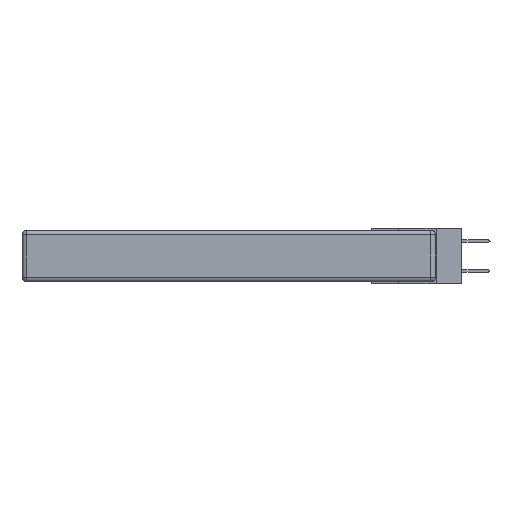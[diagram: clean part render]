
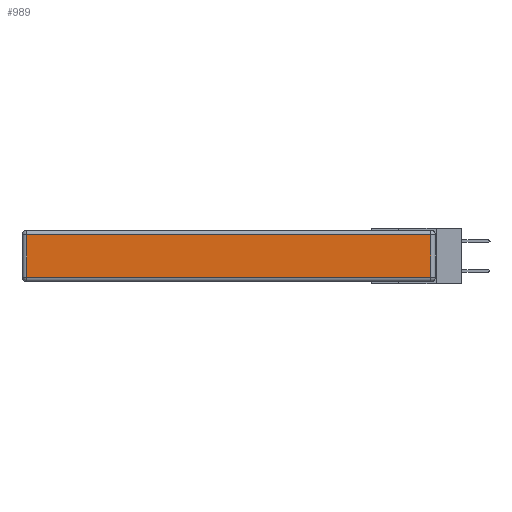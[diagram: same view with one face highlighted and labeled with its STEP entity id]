
A CAD part, left-side view. The second image highlights one B-rep face of the part: STEP entity #989.
In plain terms, the highlighted planar face has unit normal (-1, 0, 0).
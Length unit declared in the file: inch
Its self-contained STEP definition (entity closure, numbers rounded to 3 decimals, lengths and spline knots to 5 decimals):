
#612 = EDGE_CURVE ( 'NONE', #9222, #27523, #4498, .T. ) ;
#835 = CARTESIAN_POINT ( 'NONE',  ( 0., 0., -0.343 ) ) ;
#989 = ADVANCED_FACE ( 'NONE', ( #16311 ), #11534, .T. ) ;
#2759 = CARTESIAN_POINT ( 'NONE',  ( 0., 0., -0.313 ) ) ;
#4498 = LINE ( 'NONE', #10160, #17363 ) ;
#4716 = ORIENTED_EDGE ( 'NONE', *, *, #22027, .T. ) ;
#5216 = DIRECTION ( 'NONE',  ( 0., 0., 1. ) ) ;
#5951 = ORIENTED_EDGE ( 'NONE', *, *, #17439, .T. ) ;
#5953 = CARTESIAN_POINT ( 'NONE',  ( 0., 0.03, -0.03 ) ) ;
#6062 = CARTESIAN_POINT ( 'NONE',  ( 0., 2.75, -0.03 ) ) ;
#6130 = DIRECTION ( 'NONE',  ( 0., 0., 1. ) ) ;
#7300 = CARTESIAN_POINT ( 'NONE',  ( 0., 0.03, -0.313 ) ) ;
#7543 = VECTOR ( 'NONE', #14120, 39.37008 ) ;
#8411 = CARTESIAN_POINT ( 'NONE',  ( 0., 2.72, -0.313 ) ) ;
#8640 = EDGE_CURVE ( 'NONE', #15435, #14206, #14609, .T. ) ;
#8843 = VECTOR ( 'NONE', #10572, 39.37008 ) ;
#9222 = VERTEX_POINT ( 'NONE', #7300 ) ;
#9457 = LINE ( 'NONE', #2759, #16567 ) ;
#10160 = CARTESIAN_POINT ( 'NONE',  ( 0., 0.03, -0.343 ) ) ;
#10572 = DIRECTION ( 'NONE',  ( 0., 1., 0. ) ) ;
#11446 = ORIENTED_EDGE ( 'NONE', *, *, #612, .T. ) ;
#11534 = PLANE ( 'NONE',  #17292 ) ;
#11730 = DIRECTION ( 'NONE',  ( -1., 0., 0. ) ) ;
#11951 = CARTESIAN_POINT ( 'NONE',  ( 0., 2.72, -0.343 ) ) ;
#14120 = DIRECTION ( 'NONE',  ( 0., 0., -1. ) ) ;
#14206 = VERTEX_POINT ( 'NONE', #8411 ) ;
#14609 = LINE ( 'NONE', #11951, #7543 ) ;
#15435 = VERTEX_POINT ( 'NONE', #22538 ) ;
#16311 = FACE_OUTER_BOUND ( 'NONE', #19851, .T. ) ;
#16567 = VECTOR ( 'NONE', #26714, 39.37008 ) ;
#17292 = AXIS2_PLACEMENT_3D ( 'NONE', #835, #11730, #5216 ) ;
#17363 = VECTOR ( 'NONE', #6130, 39.37008 ) ;
#17439 = EDGE_CURVE ( 'NONE', #14206, #9222, #9457, .T. ) ;
#19851 = EDGE_LOOP ( 'NONE', ( #5951, #11446, #4716, #22707 ) ) ;
#20323 = LINE ( 'NONE', #6062, #8843 ) ;
#22027 = EDGE_CURVE ( 'NONE', #27523, #15435, #20323, .T. ) ;
#22538 = CARTESIAN_POINT ( 'NONE',  ( 0., 2.72, -0.03 ) ) ;
#22707 = ORIENTED_EDGE ( 'NONE', *, *, #8640, .T. ) ;
#26714 = DIRECTION ( 'NONE',  ( 0., -1., 0. ) ) ;
#27523 = VERTEX_POINT ( 'NONE', #5953 ) ;
